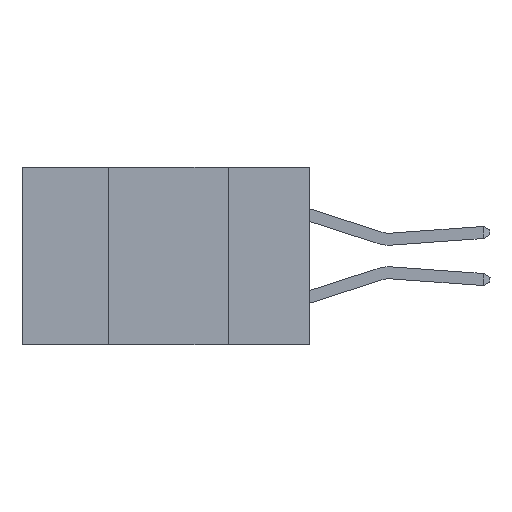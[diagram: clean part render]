
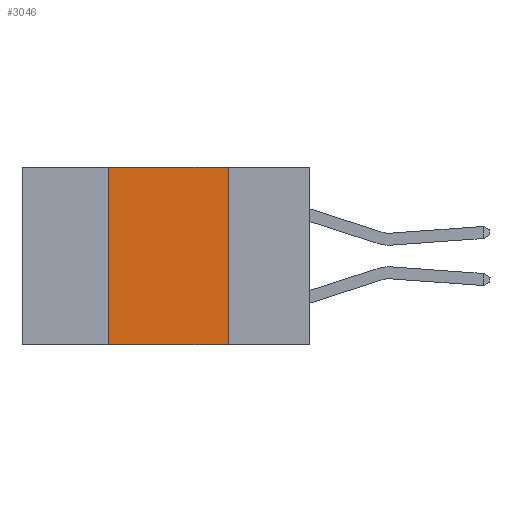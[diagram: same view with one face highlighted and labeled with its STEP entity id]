
A CAD part, left-side view. The second image highlights one B-rep face of the part: STEP entity #3046.
In plain terms, the highlighted planar face has unit normal (-1, 0, 0).
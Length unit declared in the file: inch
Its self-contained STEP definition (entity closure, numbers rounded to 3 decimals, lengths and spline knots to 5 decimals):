
#909 = DIRECTION ( 'NONE',  ( 1., 0., 0. ) ) ;
#1108 = VECTOR ( 'NONE', #14491, 39.37008 ) ;
#1407 = CARTESIAN_POINT ( 'NONE',  ( 0., 0.42, 0. ) ) ;
#2510 = ORIENTED_EDGE ( 'NONE', *, *, #9909, .T. ) ;
#2519 = CARTESIAN_POINT ( 'NONE',  ( 0., 0.42, 0. ) ) ;
#3046 = ADVANCED_FACE ( 'NONE', ( #8445 ), #5449, .F. ) ;
#4809 = VERTEX_POINT ( 'NONE', #10171 ) ;
#5449 = PLANE ( 'NONE',  #7094 ) ;
#5896 = EDGE_LOOP ( 'NONE', ( #6141, #10885, #10173, #2510 ) ) ;
#6141 = ORIENTED_EDGE ( 'NONE', *, *, #6253, .F. ) ;
#6253 = EDGE_CURVE ( 'NONE', #4809, #12502, #13870, .T. ) ;
#7094 = AXIS2_PLACEMENT_3D ( 'NONE', #11393, #909, #9112 ) ;
#7235 = DIRECTION ( 'NONE',  ( 0., -1., 0. ) ) ;
#7370 = CARTESIAN_POINT ( 'NONE',  ( 0., 0.17, 0. ) ) ;
#7756 = LINE ( 'NONE', #2519, #11282 ) ;
#8053 = VERTEX_POINT ( 'NONE', #1407 ) ;
#8059 = VERTEX_POINT ( 'NONE', #8612 ) ;
#8335 = DIRECTION ( 'NONE',  ( 0., -1., 0. ) ) ;
#8445 = FACE_OUTER_BOUND ( 'NONE', #5896, .T. ) ;
#8612 = CARTESIAN_POINT ( 'NONE',  ( 0., 0.42, -0.37 ) ) ;
#8796 = EDGE_CURVE ( 'NONE', #8053, #4809, #9002, .T. ) ;
#9002 = LINE ( 'NONE', #11962, #11051 ) ;
#9112 = DIRECTION ( 'NONE',  ( 0., 0., -1. ) ) ;
#9909 = EDGE_CURVE ( 'NONE', #8059, #12502, #13177, .T. ) ;
#10171 = CARTESIAN_POINT ( 'NONE',  ( 0., 0.17, 0. ) ) ;
#10173 = ORIENTED_EDGE ( 'NONE', *, *, #13049, .F. ) ;
#10885 = ORIENTED_EDGE ( 'NONE', *, *, #8796, .F. ) ;
#10989 = DIRECTION ( 'NONE',  ( 0., 0., 1. ) ) ;
#11051 = VECTOR ( 'NONE', #8335, 39.37008 ) ;
#11282 = VECTOR ( 'NONE', #10989, 39.37008 ) ;
#11393 = CARTESIAN_POINT ( 'NONE',  ( 0., 0.6, 0. ) ) ;
#11962 = CARTESIAN_POINT ( 'NONE',  ( 0., 0.6, 0. ) ) ;
#12502 = VERTEX_POINT ( 'NONE', #12942 ) ;
#12942 = CARTESIAN_POINT ( 'NONE',  ( 0., 0.17, -0.37 ) ) ;
#13049 = EDGE_CURVE ( 'NONE', #8059, #8053, #7756, .T. ) ;
#13177 = LINE ( 'NONE', #14294, #13546 ) ;
#13546 = VECTOR ( 'NONE', #7235, 39.37008 ) ;
#13870 = LINE ( 'NONE', #7370, #1108 ) ;
#14294 = CARTESIAN_POINT ( 'NONE',  ( 0., 0.6, -0.37 ) ) ;
#14491 = DIRECTION ( 'NONE',  ( 0., 0., -1. ) ) ;
